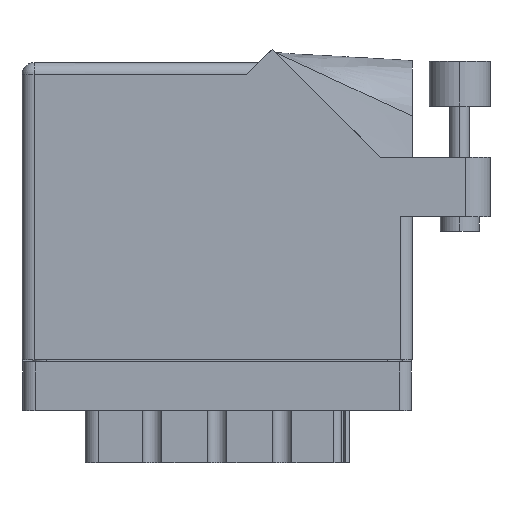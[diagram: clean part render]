
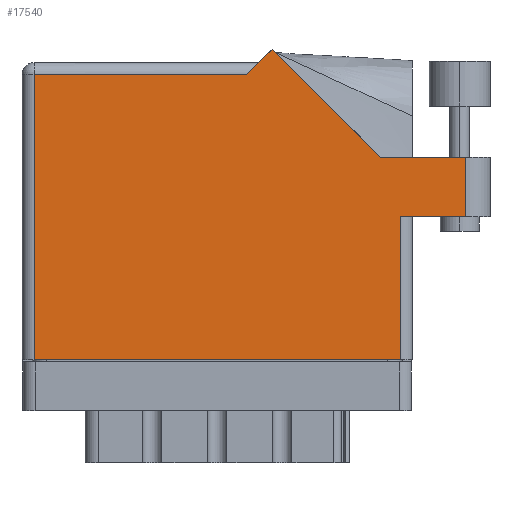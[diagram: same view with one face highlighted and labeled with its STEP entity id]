
A CAD part, front view. The second image highlights one B-rep face of the part: STEP entity #17540.
In plain terms, the highlighted face is planar.
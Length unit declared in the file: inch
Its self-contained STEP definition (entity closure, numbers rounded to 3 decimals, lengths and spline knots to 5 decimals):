
#67 = PLANE ( 'NONE',  #2858 ) ;
#424 = CARTESIAN_POINT ( 'NONE',  ( 0.062, 0., 0. ) ) ;
#1115 = LINE ( 'NONE', #21710, #10668 ) ;
#2197 = CARTESIAN_POINT ( 'NONE',  ( 2.285, 0.737, 0. ) ) ;
#2570 = DIRECTION ( 'NONE',  ( 0., 0., -1. ) ) ;
#2858 = AXIS2_PLACEMENT_3D ( 'NONE', #40928, #2570, #34470 ) ;
#4417 = EDGE_CURVE ( 'NONE', #4925, #16238, #4879, .T. ) ;
#4879 = LINE ( 'NONE', #15947, #20359 ) ;
#4925 = VERTEX_POINT ( 'NONE', #424 ) ;
#5037 = CARTESIAN_POINT ( 'NONE',  ( 1.948, 0., 0. ) ) ;
#5704 = CARTESIAN_POINT ( 'NONE',  ( 1.84442, 1.044, 0. ) ) ;
#6517 = CARTESIAN_POINT ( 'NONE',  ( 1.28771, 1.60071, 0. ) ) ;
#7010 = VERTEX_POINT ( 'NONE', #2197 ) ;
#7527 = CARTESIAN_POINT ( 'NONE',  ( 1.84442, 1.044, 0. ) ) ;
#8398 = CARTESIAN_POINT ( 'NONE',  ( 2.285, 1.044, 0. ) ) ;
#8452 = LINE ( 'NONE', #37149, #15375 ) ;
#8747 = DIRECTION ( 'NONE',  ( 0., 1., 0. ) ) ;
#9245 = VERTEX_POINT ( 'NONE', #25036 ) ;
#10332 = EDGE_CURVE ( 'NONE', #17057, #33698, #8452, .T. ) ;
#10668 = VECTOR ( 'NONE', #8747, 39.37008 ) ;
#11305 = ORIENTED_EDGE ( 'NONE', *, *, #41110, .T. ) ;
#12514 = VERTEX_POINT ( 'NONE', #39626 ) ;
#12689 = CARTESIAN_POINT ( 'NONE',  ( 2.41, 1.044, 0. ) ) ;
#13329 = EDGE_CURVE ( 'NONE', #7010, #32082, #30718, .T. ) ;
#13390 = DIRECTION ( 'NONE',  ( 1., 0., 0. ) ) ;
#14665 = ORIENTED_EDGE ( 'NONE', *, *, #29835, .T. ) ;
#15095 = DIRECTION ( 'NONE',  ( -0.707, 0.707, 0. ) ) ;
#15375 = VECTOR ( 'NONE', #30299, 39.37008 ) ;
#15880 = VECTOR ( 'NONE', #36212, 39.37008 ) ;
#15947 = CARTESIAN_POINT ( 'NONE',  ( 0., 0., 0. ) ) ;
#16090 = VECTOR ( 'NONE', #40539, 39.37008 ) ;
#16238 = VERTEX_POINT ( 'NONE', #5037 ) ;
#16370 = EDGE_CURVE ( 'NONE', #22430, #17057, #20057, .T. ) ;
#17057 = VERTEX_POINT ( 'NONE', #6517 ) ;
#17067 = ORIENTED_EDGE ( 'NONE', *, *, #21328, .T. ) ;
#17242 = VECTOR ( 'NONE', #24435, 39.37008 ) ;
#17333 = VECTOR ( 'NONE', #35102, 39.37008 ) ;
#17540 = ADVANCED_FACE ( 'NONE', ( #19676 ), #67, .F. ) ;
#17571 = VECTOR ( 'NONE', #15095, 39.37008 ) ;
#18091 = ORIENTED_EDGE ( 'NONE', *, *, #41078, .T. ) ;
#18990 = DIRECTION ( 'NONE',  ( 1., 0., 0. ) ) ;
#19676 = FACE_OUTER_BOUND ( 'NONE', #32599, .T. ) ;
#20057 = LINE ( 'NONE', #5704, #17571 ) ;
#20359 = VECTOR ( 'NONE', #18990, 39.37008 ) ;
#20503 = ORIENTED_EDGE ( 'NONE', *, *, #31708, .T. ) ;
#21287 = CARTESIAN_POINT ( 'NONE',  ( 0., 1.468, 0. ) ) ;
#21328 = EDGE_CURVE ( 'NONE', #9245, #7010, #36388, .T. ) ;
#21710 = CARTESIAN_POINT ( 'NONE',  ( 1.948, 0.737, 0. ) ) ;
#21827 = CARTESIAN_POINT ( 'NONE',  ( 1.155, 1.468, 0. ) ) ;
#22376 = LINE ( 'NONE', #21287, #15880 ) ;
#22430 = VERTEX_POINT ( 'NONE', #7527 ) ;
#22853 = CARTESIAN_POINT ( 'NONE',  ( 2.01, 0.737, 0. ) ) ;
#24435 = DIRECTION ( 'NONE',  ( 0., 1., 0. ) ) ;
#25035 = CARTESIAN_POINT ( 'NONE',  ( 0.062, 0., 0. ) ) ;
#25036 = CARTESIAN_POINT ( 'NONE',  ( 1.948, 0.737, 0. ) ) ;
#26031 = ORIENTED_EDGE ( 'NONE', *, *, #16370, .T. ) ;
#28550 = ORIENTED_EDGE ( 'NONE', *, *, #10332, .T. ) ;
#28624 = ORIENTED_EDGE ( 'NONE', *, *, #13329, .T. ) ;
#28896 = VECTOR ( 'NONE', #13390, 39.37008 ) ;
#29835 = EDGE_CURVE ( 'NONE', #33698, #12514, #22376, .T. ) ;
#30299 = DIRECTION ( 'NONE',  ( -0.707, -0.707, 0. ) ) ;
#30718 = LINE ( 'NONE', #8398, #17242 ) ;
#31708 = EDGE_CURVE ( 'NONE', #32082, #22430, #38735, .T. ) ;
#32082 = VERTEX_POINT ( 'NONE', #38834 ) ;
#32599 = EDGE_LOOP ( 'NONE', ( #17067, #28624, #20503, #26031, #28550, #14665, #18091, #34636, #11305 ) ) ;
#33698 = VERTEX_POINT ( 'NONE', #21827 ) ;
#34470 = DIRECTION ( 'NONE',  ( -1., 0., 0. ) ) ;
#34636 = ORIENTED_EDGE ( 'NONE', *, *, #4417, .T. ) ;
#35102 = DIRECTION ( 'NONE',  ( -1., 0., 0. ) ) ;
#36212 = DIRECTION ( 'NONE',  ( -1., 0., 0. ) ) ;
#36388 = LINE ( 'NONE', #22853, #28896 ) ;
#37149 = CARTESIAN_POINT ( 'NONE',  ( 1.217, 1.53, 0. ) ) ;
#38033 = LINE ( 'NONE', #25035, #16090 ) ;
#38735 = LINE ( 'NONE', #12689, #17333 ) ;
#38834 = CARTESIAN_POINT ( 'NONE',  ( 2.285, 1.044, 0. ) ) ;
#39626 = CARTESIAN_POINT ( 'NONE',  ( 0.062, 1.468, 0. ) ) ;
#40539 = DIRECTION ( 'NONE',  ( 0., -1., 0. ) ) ;
#40928 = CARTESIAN_POINT ( 'NONE',  ( 0., 1.53, 0. ) ) ;
#41078 = EDGE_CURVE ( 'NONE', #12514, #4925, #38033, .T. ) ;
#41110 = EDGE_CURVE ( 'NONE', #16238, #9245, #1115, .T. ) ;
